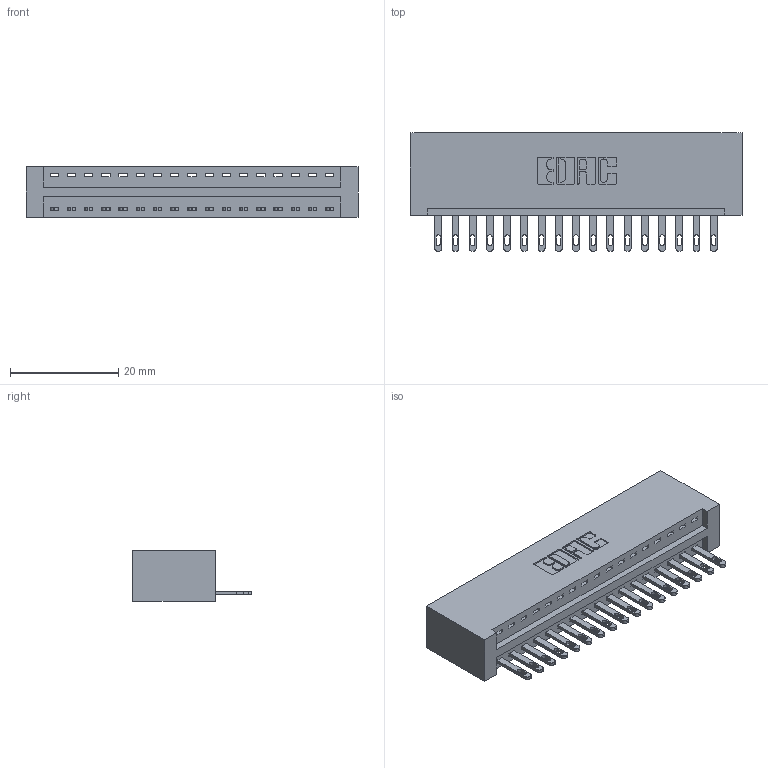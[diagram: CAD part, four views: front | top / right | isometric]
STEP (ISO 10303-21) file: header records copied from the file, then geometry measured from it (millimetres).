
FILE_DESCRIPTION (( 'STEP AP203' ), '1' );
FILE_NAME ('896-017-500-101.STEP', '2021-07-27T15:49:50', ( '' ), ( '' ), 'SwSTEP 2.0', 'SolidWorks 2020', '' );
FILE_SCHEMA (( 'CONFIG_CONTROL_DESIGN' ));
Length unit declared in the file: inch
Products named in the file (3): 846 Part_No Mounting Lugs; 345-292-001_345-293-100; 896-017-500-101
Assembly tree (18 placements, depth 2):
  896-017-500-101
    846 Part_No Mounting Lugs
    345-292-001_345-293-100  x17
Bounding box: 61.21 x 21.84 x 9.4 mm (x, y, z)
Volume: 6247.2 mm3; surface area: 7653.2 mm2
Topology: 18 solids, 18 shells, 1032 faces, 3161 edges, 2106 vertices
Faces by surface type: plane 650, cylinder 382
Entity records: 13569 total; most frequent: CARTESIAN_POINT 2339, ORIENTED_EDGE 2290, DIRECTION 2091, EDGE_CURVE 1145, VECTOR 949, LINE 949, VERTEX_POINT 762, AXIS2_PLACEMENT_3D 571
